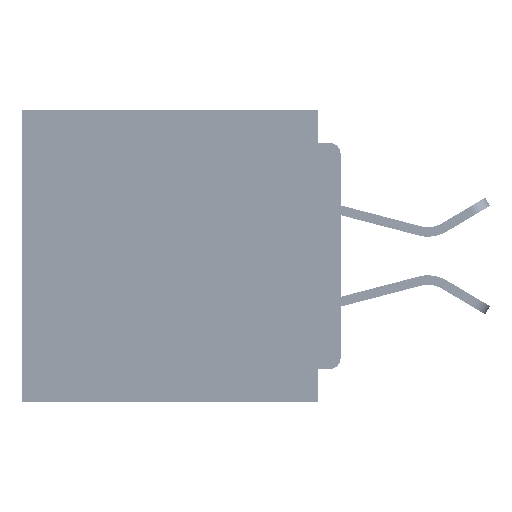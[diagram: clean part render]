
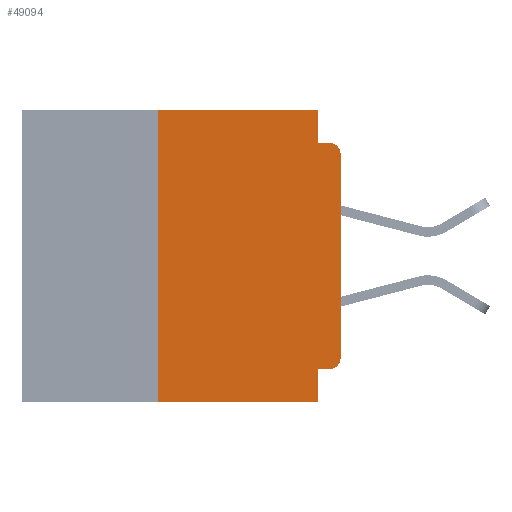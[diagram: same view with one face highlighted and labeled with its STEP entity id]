
A CAD part, left-side view. The second image highlights one B-rep face of the part: STEP entity #49094.
In plain terms, the highlighted planar face has unit normal (-1, 0, 0).
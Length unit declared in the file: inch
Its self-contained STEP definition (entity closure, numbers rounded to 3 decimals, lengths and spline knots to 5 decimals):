
#427 = CARTESIAN_POINT ( 'NONE',  ( 0., 0.031, -0.045 ) ) ;
#2292 = EDGE_CURVE ( 'NONE', #56660, #23437, #31913, .T. ) ;
#2575 = VERTEX_POINT ( 'NONE', #34167 ) ;
#3136 = VECTOR ( 'NONE', #32652, 39.37008 ) ;
#3338 = CARTESIAN_POINT ( 'NONE',  ( 0., 0.015, -0.34 ) ) ;
#3883 = VECTOR ( 'NONE', #3978, 39.37008 ) ;
#3978 = DIRECTION ( 'NONE',  ( 0., -1., 0. ) ) ;
#4192 = CARTESIAN_POINT ( 'NONE',  ( 0., 0.031, 0. ) ) ;
#4469 = CIRCLE ( 'NONE', #50670, 0.015 ) ;
#4617 = VERTEX_POINT ( 'NONE', #14771 ) ;
#6282 = EDGE_CURVE ( 'NONE', #2575, #40174, #14298, .T. ) ;
#6740 = EDGE_CURVE ( 'NONE', #20423, #38838, #25350, .T. ) ;
#7733 = VECTOR ( 'NONE', #24856, 39.37008 ) ;
#8102 = DIRECTION ( 'NONE',  ( 0., 0., -1. ) ) ;
#8297 = PLANE ( 'NONE',  #43761 ) ;
#10412 = CARTESIAN_POINT ( 'NONE',  ( 0., 0.015, -0.355 ) ) ;
#11328 = ORIENTED_EDGE ( 'NONE', *, *, #2292, .F. ) ;
#12776 = ORIENTED_EDGE ( 'NONE', *, *, #40792, .F. ) ;
#12858 = EDGE_CURVE ( 'NONE', #4617, #35545, #27511, .T. ) ;
#13086 = DIRECTION ( 'NONE',  ( 1., 0., 0. ) ) ;
#13366 = EDGE_CURVE ( 'NONE', #16353, #20423, #49737, .T. ) ;
#13548 = EDGE_CURVE ( 'NONE', #35545, #2575, #37810, .T. ) ;
#14298 = LINE ( 'NONE', #4192, #3136 ) ;
#14771 = CARTESIAN_POINT ( 'NONE',  ( 0., 0.25, -0.4 ) ) ;
#14906 = VECTOR ( 'NONE', #55635, 39.37008 ) ;
#16283 = EDGE_LOOP ( 'NONE', ( #27589, #19466, #12776, #37991, #59478, #40263, #35090, #11328, #41041, #29889 ) ) ;
#16353 = VERTEX_POINT ( 'NONE', #55844 ) ;
#16858 = EDGE_CURVE ( 'NONE', #59775, #56660, #16913, .T. ) ;
#16913 = LINE ( 'NONE', #26135, #40643 ) ;
#17345 = CARTESIAN_POINT ( 'NONE',  ( 0., 0.015, -0.06 ) ) ;
#17725 = CARTESIAN_POINT ( 'NONE',  ( 0., 0.25, -0.4 ) ) ;
#19466 = ORIENTED_EDGE ( 'NONE', *, *, #6740, .T. ) ;
#20423 = VERTEX_POINT ( 'NONE', #35254 ) ;
#21803 = CARTESIAN_POINT ( 'NONE',  ( 0., 0.031, -0.4 ) ) ;
#22127 = DIRECTION ( 'NONE',  ( 0., 0., -1. ) ) ;
#23437 = VERTEX_POINT ( 'NONE', #21803 ) ;
#24856 = DIRECTION ( 'NONE',  ( 0., -1., 0. ) ) ;
#25350 = CIRCLE ( 'NONE', #58811, 0.015 ) ;
#26135 = CARTESIAN_POINT ( 'NONE',  ( 0., 0., -0.355 ) ) ;
#26320 = CARTESIAN_POINT ( 'NONE',  ( 0., 0., 0. ) ) ;
#27511 = LINE ( 'NONE', #17725, #14906 ) ;
#27589 = ORIENTED_EDGE ( 'NONE', *, *, #13366, .T. ) ;
#27646 = CARTESIAN_POINT ( 'NONE',  ( 0., 0.437, -0.4 ) ) ;
#29439 = EDGE_CURVE ( 'NONE', #59775, #16353, #4469, .T. ) ;
#29889 = ORIENTED_EDGE ( 'NONE', *, *, #29439, .T. ) ;
#30627 = LINE ( 'NONE', #27646, #3883 ) ;
#31365 = FACE_OUTER_BOUND ( 'NONE', #16283, .T. ) ;
#31913 = LINE ( 'NONE', #44415, #40050 ) ;
#32340 = DIRECTION ( 'NONE',  ( 0., -1., 0. ) ) ;
#32652 = DIRECTION ( 'NONE',  ( 0., 0., -1. ) ) ;
#33798 = EDGE_CURVE ( 'NONE', #4617, #23437, #30627, .T. ) ;
#34167 = CARTESIAN_POINT ( 'NONE',  ( 0., 0.031, 0. ) ) ;
#35090 = ORIENTED_EDGE ( 'NONE', *, *, #33798, .T. ) ;
#35254 = CARTESIAN_POINT ( 'NONE',  ( 0., 0., -0.06 ) ) ;
#35545 = VERTEX_POINT ( 'NONE', #46348 ) ;
#36529 = DIRECTION ( 'NONE',  ( -1., 0., 0. ) ) ;
#37093 = CARTESIAN_POINT ( 'NONE',  ( 0., 0.437, 0. ) ) ;
#37810 = LINE ( 'NONE', #37093, #48960 ) ;
#37991 = ORIENTED_EDGE ( 'NONE', *, *, #6282, .F. ) ;
#38838 = VERTEX_POINT ( 'NONE', #47698 ) ;
#40050 = VECTOR ( 'NONE', #43700, 39.37008 ) ;
#40174 = VERTEX_POINT ( 'NONE', #427 ) ;
#40263 = ORIENTED_EDGE ( 'NONE', *, *, #12858, .F. ) ;
#40643 = VECTOR ( 'NONE', #50009, 39.37008 ) ;
#40792 = EDGE_CURVE ( 'NONE', #40174, #38838, #45599, .T. ) ;
#41041 = ORIENTED_EDGE ( 'NONE', *, *, #16858, .F. ) ;
#43700 = DIRECTION ( 'NONE',  ( 0., 0., -1. ) ) ;
#43761 = AXIS2_PLACEMENT_3D ( 'NONE', #60297, #13086, #46284 ) ;
#44415 = CARTESIAN_POINT ( 'NONE',  ( 0., 0.031, -0.4 ) ) ;
#44738 = CARTESIAN_POINT ( 'NONE',  ( 0., 0.031, -0.355 ) ) ;
#45599 = LINE ( 'NONE', #53304, #7733 ) ;
#46284 = DIRECTION ( 'NONE',  ( 0., 0., -1. ) ) ;
#46348 = CARTESIAN_POINT ( 'NONE',  ( 0., 0.25, 0. ) ) ;
#47698 = CARTESIAN_POINT ( 'NONE',  ( 0., 0.015, -0.045 ) ) ;
#48960 = VECTOR ( 'NONE', #32340, 39.37008 ) ;
#49094 = ADVANCED_FACE ( 'NONE', ( #31365 ), #8297, .F. ) ;
#49737 = LINE ( 'NONE', #26320, #60777 ) ;
#50009 = DIRECTION ( 'NONE',  ( 0., 1., 0. ) ) ;
#50524 = DIRECTION ( 'NONE',  ( -1., 0., 0. ) ) ;
#50670 = AXIS2_PLACEMENT_3D ( 'NONE', #3338, #36529, #8102 ) ;
#53304 = CARTESIAN_POINT ( 'NONE',  ( 0., 0., -0.045 ) ) ;
#54744 = DIRECTION ( 'NONE',  ( 0., 0., 1. ) ) ;
#55635 = DIRECTION ( 'NONE',  ( 0., 0., 1. ) ) ;
#55844 = CARTESIAN_POINT ( 'NONE',  ( 0., 0., -0.34 ) ) ;
#56660 = VERTEX_POINT ( 'NONE', #44738 ) ;
#58811 = AXIS2_PLACEMENT_3D ( 'NONE', #17345, #50524, #22127 ) ;
#59478 = ORIENTED_EDGE ( 'NONE', *, *, #13548, .F. ) ;
#59775 = VERTEX_POINT ( 'NONE', #10412 ) ;
#60297 = CARTESIAN_POINT ( 'NONE',  ( 0., 0.437, 0. ) ) ;
#60777 = VECTOR ( 'NONE', #54744, 39.37008 ) ;
